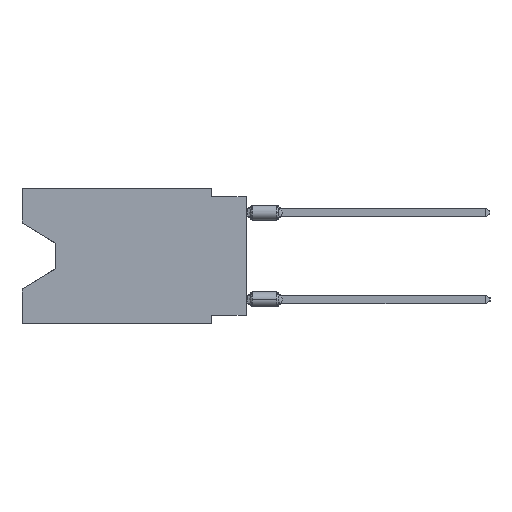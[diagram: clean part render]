
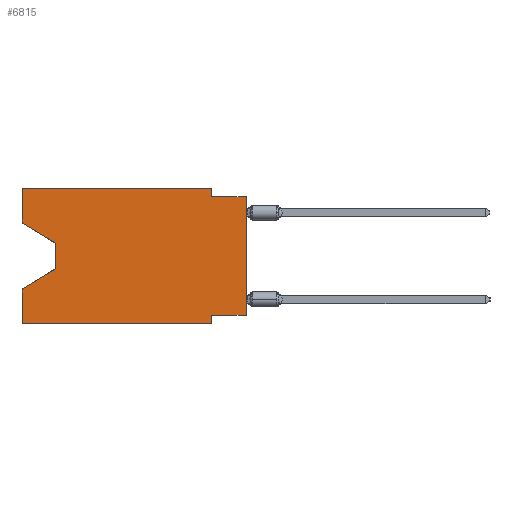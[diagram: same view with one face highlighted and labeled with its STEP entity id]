
A CAD part, left-side view. The second image highlights one B-rep face of the part: STEP entity #6815.
In plain terms, the highlighted planar face has unit normal (-1, 0, 0).
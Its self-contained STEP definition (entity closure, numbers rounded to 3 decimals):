
#350 = CARTESIAN_POINT ( 'NONE',  ( 0., 16.383, 0. ) ) ;
#1032 = VECTOR ( 'NONE', #49760, 1000. ) ;
#1069 = VERTEX_POINT ( 'NONE', #10013 ) ;
#1409 = EDGE_CURVE ( 'NONE', #1069, #23341, #36860, .T. ) ;
#1772 = VECTOR ( 'NONE', #53896, 1000. ) ;
#2858 = DIRECTION ( 'NONE',  ( 0., -1., 0. ) ) ;
#3152 = DIRECTION ( 'NONE',  ( 0., 0., 1. ) ) ;
#3960 = FACE_OUTER_BOUND ( 'NONE', #20501, .T. ) ;
#5159 = LINE ( 'NONE', #23437, #35871 ) ;
#5182 = LINE ( 'NONE', #6879, #33773 ) ;
#5195 = CARTESIAN_POINT ( 'NONE',  ( 0., 13.97, -5.893 ) ) ;
#5902 = VERTEX_POINT ( 'NONE', #50136 ) ;
#6815 = ADVANCED_FACE ( 'NONE', ( #3960 ), #23111, .F. ) ;
#6879 = CARTESIAN_POINT ( 'NONE',  ( 0., 16.383, -9.906 ) ) ;
#7166 = EDGE_CURVE ( 'NONE', #29449, #35118, #23861, .T. ) ;
#7216 = EDGE_CURVE ( 'NONE', #43516, #56724, #25331, .T. ) ;
#7653 = LINE ( 'NONE', #44209, #20595 ) ;
#8554 = VECTOR ( 'NONE', #24367, 1000. ) ;
#10013 = CARTESIAN_POINT ( 'NONE',  ( 0., 2.54, -0.635 ) ) ;
#11325 = DIRECTION ( 'NONE',  ( 0., 0., 1. ) ) ;
#11834 = LINE ( 'NONE', #30134, #50353 ) ;
#13004 = VERTEX_POINT ( 'NONE', #54304 ) ;
#13439 = CARTESIAN_POINT ( 'NONE',  ( 0., 2.54, 0. ) ) ;
#13844 = DIRECTION ( 'NONE',  ( 0., -0.855, -0.519 ) ) ;
#14648 = VERTEX_POINT ( 'NONE', #22659 ) ;
#15137 = EDGE_CURVE ( 'NONE', #35118, #13004, #33060, .T. ) ;
#15487 = ORIENTED_EDGE ( 'NONE', *, *, #52944, .T. ) ;
#16471 = CARTESIAN_POINT ( 'NONE',  ( 0., 2.54, -9.271 ) ) ;
#19070 = DIRECTION ( 'NONE',  ( 0., 0., -1. ) ) ;
#20167 = DIRECTION ( 'NONE',  ( 0., 0., 1. ) ) ;
#20247 = CARTESIAN_POINT ( 'NONE',  ( 0., 0., -0.635 ) ) ;
#20501 = EDGE_LOOP ( 'NONE', ( #15487, #25341, #31707, #54272, #30809, #44680, #28154, #21943, #53429, #50560, #57064, #39284 ) ) ;
#20595 = VECTOR ( 'NONE', #3152, 1000. ) ;
#21943 = ORIENTED_EDGE ( 'NONE', *, *, #48248, .T. ) ;
#22418 = LINE ( 'NONE', #13439, #1772 ) ;
#22546 = CARTESIAN_POINT ( 'NONE',  ( 0., 13.97, -5.893 ) ) ;
#22659 = CARTESIAN_POINT ( 'NONE',  ( 0., 0., -9.271 ) ) ;
#22837 = VERTEX_POINT ( 'NONE', #32333 ) ;
#23111 = PLANE ( 'NONE',  #53177 ) ;
#23341 = VERTEX_POINT ( 'NONE', #20247 ) ;
#23437 = CARTESIAN_POINT ( 'NONE',  ( 0., 16.383, -2.546 ) ) ;
#23861 = LINE ( 'NONE', #55910, #55099 ) ;
#24367 = DIRECTION ( 'NONE',  ( 0., 0.855, -0.519 ) ) ;
#24840 = EDGE_CURVE ( 'NONE', #25256, #39728, #11834, .T. ) ;
#24878 = DIRECTION ( 'NONE',  ( 0., -1., 0. ) ) ;
#25042 = CARTESIAN_POINT ( 'NONE',  ( 0., 2.54, -9.906 ) ) ;
#25256 = VERTEX_POINT ( 'NONE', #350 ) ;
#25331 = LINE ( 'NONE', #25042, #58020 ) ;
#25341 = ORIENTED_EDGE ( 'NONE', *, *, #7166, .T. ) ;
#28154 = ORIENTED_EDGE ( 'NONE', *, *, #47962, .F. ) ;
#29244 = EDGE_CURVE ( 'NONE', #39728, #1069, #22418, .T. ) ;
#29449 = VERTEX_POINT ( 'NONE', #48455 ) ;
#30089 = CARTESIAN_POINT ( 'NONE',  ( 0., 2.54, 0. ) ) ;
#30134 = CARTESIAN_POINT ( 'NONE',  ( 0., 16.383, 0. ) ) ;
#30809 = ORIENTED_EDGE ( 'NONE', *, *, #56123, .T. ) ;
#31707 = ORIENTED_EDGE ( 'NONE', *, *, #15137, .T. ) ;
#32333 = CARTESIAN_POINT ( 'NONE',  ( 0., 16.383, -2.546 ) ) ;
#33060 = LINE ( 'NONE', #5195, #8554 ) ;
#33773 = VECTOR ( 'NONE', #24878, 1000. ) ;
#34106 = LINE ( 'NONE', #52381, #52879 ) ;
#35118 = VERTEX_POINT ( 'NONE', #22546 ) ;
#35871 = VECTOR ( 'NONE', #13844, 1000. ) ;
#36532 = CARTESIAN_POINT ( 'NONE',  ( 0., 0., -9.271 ) ) ;
#36860 = LINE ( 'NONE', #55409, #1032 ) ;
#39284 = ORIENTED_EDGE ( 'NONE', *, *, #47836, .F. ) ;
#39728 = VERTEX_POINT ( 'NONE', #30089 ) ;
#41696 = DIRECTION ( 'NONE',  ( 0., 0., -1. ) ) ;
#43516 = VERTEX_POINT ( 'NONE', #16471 ) ;
#44209 = CARTESIAN_POINT ( 'NONE',  ( 0., 16.383, 0. ) ) ;
#44680 = ORIENTED_EDGE ( 'NONE', *, *, #7216, .F. ) ;
#45198 = VECTOR ( 'NONE', #59000, 1000. ) ;
#45812 = LINE ( 'NONE', #36532, #45198 ) ;
#47836 = EDGE_CURVE ( 'NONE', #22837, #25256, #57309, .T. ) ;
#47962 = EDGE_CURVE ( 'NONE', #14648, #43516, #45812, .T. ) ;
#48248 = EDGE_CURVE ( 'NONE', #14648, #23341, #34106, .T. ) ;
#48455 = CARTESIAN_POINT ( 'NONE',  ( 0., 13.97, -4.013 ) ) ;
#49515 = DIRECTION ( 'NONE',  ( 1., 0., 0. ) ) ;
#49760 = DIRECTION ( 'NONE',  ( 0., -1., 0. ) ) ;
#50136 = CARTESIAN_POINT ( 'NONE',  ( 0., 16.383, -9.906 ) ) ;
#50353 = VECTOR ( 'NONE', #2858, 1000. ) ;
#50560 = ORIENTED_EDGE ( 'NONE', *, *, #29244, .F. ) ;
#50689 = CARTESIAN_POINT ( 'NONE',  ( 0., 16.383, 0. ) ) ;
#51201 = EDGE_CURVE ( 'NONE', #5902, #13004, #7653, .T. ) ;
#51634 = CARTESIAN_POINT ( 'NONE',  ( 0., 16.383, 0. ) ) ;
#52018 = DIRECTION ( 'NONE',  ( 0., 0., -1. ) ) ;
#52381 = CARTESIAN_POINT ( 'NONE',  ( 0., 0., 0. ) ) ;
#52879 = VECTOR ( 'NONE', #11325, 1000. ) ;
#52944 = EDGE_CURVE ( 'NONE', #22837, #29449, #5159, .T. ) ;
#53177 = AXIS2_PLACEMENT_3D ( 'NONE', #50689, #49515, #41696 ) ;
#53429 = ORIENTED_EDGE ( 'NONE', *, *, #1409, .F. ) ;
#53896 = DIRECTION ( 'NONE',  ( 0., 0., -1. ) ) ;
#54272 = ORIENTED_EDGE ( 'NONE', *, *, #51201, .F. ) ;
#54304 = CARTESIAN_POINT ( 'NONE',  ( 0., 16.383, -7.36 ) ) ;
#55099 = VECTOR ( 'NONE', #19070, 1000. ) ;
#55409 = CARTESIAN_POINT ( 'NONE',  ( 0., 0., -0.635 ) ) ;
#55700 = VECTOR ( 'NONE', #20167, 1000. ) ;
#55910 = CARTESIAN_POINT ( 'NONE',  ( 0., 13.97, -4.013 ) ) ;
#56123 = EDGE_CURVE ( 'NONE', #5902, #56724, #5182, .T. ) ;
#56724 = VERTEX_POINT ( 'NONE', #57731 ) ;
#57064 = ORIENTED_EDGE ( 'NONE', *, *, #24840, .F. ) ;
#57309 = LINE ( 'NONE', #51634, #55700 ) ;
#57731 = CARTESIAN_POINT ( 'NONE',  ( 0., 2.54, -9.906 ) ) ;
#58020 = VECTOR ( 'NONE', #52018, 1000. ) ;
#59000 = DIRECTION ( 'NONE',  ( 0., 1., 0. ) ) ;
